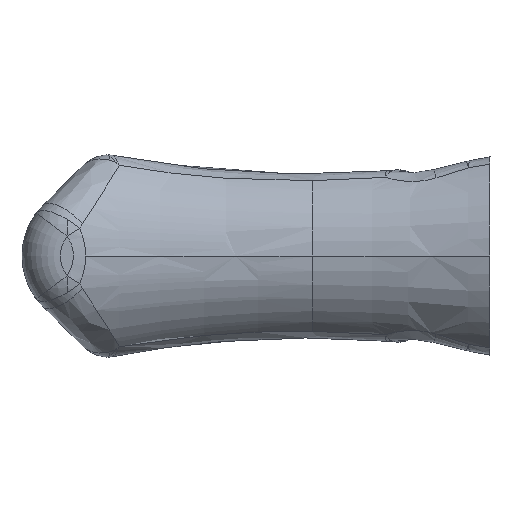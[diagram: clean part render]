
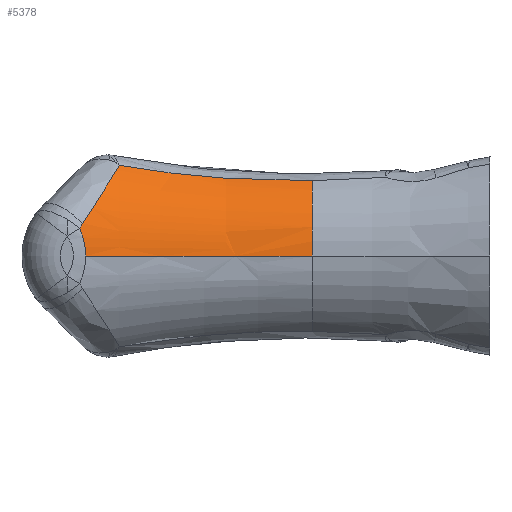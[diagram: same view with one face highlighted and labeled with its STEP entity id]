
A CAD part, left-side view. The second image highlights one B-rep face of the part: STEP entity #5378.
In plain terms, the highlighted toroidal (fillet/blend) face has major radius 208.719 mm and minor radius 185.111 mm.
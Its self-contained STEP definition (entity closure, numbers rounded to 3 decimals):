
#231 = DIRECTION ( 'NONE',  ( -1., 0., 0. ) ) ;
#347 = CARTESIAN_POINT ( 'NONE',  ( -310.696, 64.488, 25.983 ) ) ;
#418 = CARTESIAN_POINT ( 'NONE',  ( -307.871, 63.211, 28.086 ) ) ;
#647 = CARTESIAN_POINT ( 'NONE',  ( -321.046, 73.018, 12.59 ) ) ;
#705 = EDGE_CURVE ( 'NONE', #3358, #5440, #2863, .T. ) ;
#825 = CARTESIAN_POINT ( 'NONE',  ( -313.258, 65.894, 23.695 ) ) ;
#827 = B_SPLINE_CURVE_WITH_KNOTS ( 'NONE', 3,
 ( #3615, #3656, #4132, #1293, #4623, #1784, #5098, #2257 ),
 .UNSPECIFIED., .F., .F.,
 ( 4, 2, 2, 4 ),
 ( 0.011, 0.013, 0.015, 0.019 ),
 .UNSPECIFIED. ) ;
#836 = VERTEX_POINT ( 'NONE', #4522 ) ;
#878 = CARTESIAN_POINT ( 'NONE',  ( -301.785, 17.37, 24.08 ) ) ;
#899 = B_SPLINE_CURVE_WITH_KNOTS ( 'NONE', 3,
 ( #3952, #647, #4912, #2082 ),
 .UNSPECIFIED., .F., .F.,
 ( 4, 4 ),
 ( 0., 0.002 ),
 .UNSPECIFIED. ) ;
#901 = EDGE_CURVE ( 'NONE', #4754, #2436, #4038, .T. ) ;
#1188 = AXIS2_PLACEMENT_3D ( 'NONE', #5919, #3066, #231 ) ;
#1202 = EDGE_LOOP ( 'NONE', ( #6044, #1554, #4836, #1295, #6018, #1652 ) ) ;
#1293 = CARTESIAN_POINT ( 'NONE',  ( -321.548, 72.657, 9.405 ) ) ;
#1295 = ORIENTED_EDGE ( 'NONE', *, *, #901, .T. ) ;
#1296 = CARTESIAN_POINT ( 'NONE',  ( -316.564, 68.248, 19.938 ) ) ;
#1351 = CARTESIAN_POINT ( 'NONE',  ( -302.108, 23.712, 24.165 ) ) ;
#1554 = ORIENTED_EDGE ( 'NONE', *, *, #1622, .T. ) ;
#1561 = AXIS2_PLACEMENT_3D ( 'NONE', #2595, #3996, #5921 ) ;
#1622 = EDGE_CURVE ( 'NONE', #5440, #4441, #2073, .T. ) ;
#1652 = ORIENTED_EDGE ( 'NONE', *, *, #4224, .T. ) ;
#1784 = CARTESIAN_POINT ( 'NONE',  ( -321.638, 72.092, 7.004 ) ) ;
#1786 = CARTESIAN_POINT ( 'NONE',  ( -318.882, 70.421, 16.55 ) ) ;
#1838 = CARTESIAN_POINT ( 'NONE',  ( -302.604, 30.036, 24.392 ) ) ;
#1863 = CARTESIAN_POINT ( 'NONE',  ( -321.66, 71.952, 4.547 ) ) ;
#1895 = CARTESIAN_POINT ( 'NONE',  ( -301.679, 13.135, 24.108 ) ) ;
#2073 = CIRCLE ( 'NONE', #6058, 23.608 ) ;
#2082 = CARTESIAN_POINT ( 'NONE',  ( -321.417, 73.495, 11.706 ) ) ;
#2206 = CARTESIAN_POINT ( 'NONE',  ( -320.842, 72.744, 13.003 ) ) ;
#2257 = CARTESIAN_POINT ( 'NONE',  ( -321.66, 71.952, 4.547 ) ) ;
#2259 = CARTESIAN_POINT ( 'NONE',  ( -320.109, 71.798, 14.437 ) ) ;
#2266 = DIRECTION ( 'NONE',  ( 0., 1., 0. ) ) ;
#2318 = CARTESIAN_POINT ( 'NONE',  ( -303.265, 36.345, 24.763 ) ) ;
#2436 = VERTEX_POINT ( 'NONE', #2206 ) ;
#2595 = CARTESIAN_POINT ( 'NONE',  ( -288.46, 13.135, 4.547 ) ) ;
#2713 = CARTESIAN_POINT ( 'NONE',  ( -308.606, 63.511, 27.589 ) ) ;
#2734 = CARTESIAN_POINT ( 'NONE',  ( -320.842, 72.744, 13.003 ) ) ;
#2783 = CARTESIAN_POINT ( 'NONE',  ( -304.683, 46.784, 25.683 ) ) ;
#2863 = CIRCLE ( 'NONE', #1188, 185.111 ) ;
#2916 = EDGE_CURVE ( 'NONE', #2436, #836, #899, .T. ) ;
#3066 = DIRECTION ( 'NONE',  ( 0., 0., -1. ) ) ;
#3116 = FACE_OUTER_BOUND ( 'NONE', #1202, .T. ) ;
#3120 = CARTESIAN_POINT ( 'NONE',  ( -307.871, 63.211, 28.086 ) ) ;
#3192 = CARTESIAN_POINT ( 'NONE',  ( -309.319, 63.827, 27.068 ) ) ;
#3263 = CARTESIAN_POINT ( 'NONE',  ( -306.952, 59.141, 27.362 ) ) ;
#3315 = EDGE_CURVE ( 'NONE', #4441, #4754, #4394, .T. ) ;
#3358 = VERTEX_POINT ( 'NONE', #1863 ) ;
#3401 = TOROIDAL_SURFACE ( 'NONE', #1561, 208.719, 185.111 ) ;
#3615 = CARTESIAN_POINT ( 'NONE',  ( -321.417, 73.495, 11.706 ) ) ;
#3656 = CARTESIAN_POINT ( 'NONE',  ( -321.454, 73.255, 11.143 ) ) ;
#3658 = CARTESIAN_POINT ( 'NONE',  ( -311.356, 64.831, 25.423 ) ) ;
#3952 = CARTESIAN_POINT ( 'NONE',  ( -320.842, 72.744, 13.003 ) ) ;
#3996 = DIRECTION ( 'NONE',  ( 0., 1., 0. ) ) ;
#4034 = CARTESIAN_POINT ( 'NONE',  ( -312.068, 13.135, 4.547 ) ) ;
#4038 = B_SPLINE_CURVE_WITH_KNOTS ( 'NONE', 3,
 ( #6041, #2713, #3192, #347, #3658, #825, #4135, #1296, #4625, #1786, #5100, #2259, #5585, #2734 ),
 .UNSPECIFIED., .F., .F.,
 ( 4, 2, 2, 2, 2, 2, 4 ),
 ( 0., 0.003, 0.006, 0.012, 0.017, 0.02, 0.023 ),
 .UNSPECIFIED. ) ;
#4132 = CARTESIAN_POINT ( 'NONE',  ( -321.488, 73.038, 10.571 ) ) ;
#4135 = CARTESIAN_POINT ( 'NONE',  ( -314.422, 66.649, 22.479 ) ) ;
#4188 = CARTESIAN_POINT ( 'NONE',  ( -301.981, 21.6, 24.121 ) ) ;
#4224 = EDGE_CURVE ( 'NONE', #836, #3358, #827, .T. ) ;
#4394 = B_SPLINE_CURVE_WITH_KNOTS ( 'NONE', 3,
 ( #4660, #6096, #878, #4188, #1351, #4679, #1838, #5158, #2318, #5641, #2783, #6112, #3263, #418 ),
 .UNSPECIFIED., .F., .F.,
 ( 4, 2, 2, 2, 2, 2, 4 ),
 ( 0.048, 0.055, 0.061, 0.067, 0.074, 0.086, 0.099 ),
 .UNSPECIFIED. ) ;
#4441 = VERTEX_POINT ( 'NONE', #1895 ) ;
#4522 = CARTESIAN_POINT ( 'NONE',  ( -321.417, 73.495, 11.706 ) ) ;
#4623 = CARTESIAN_POINT ( 'NONE',  ( -321.575, 72.491, 8.808 ) ) ;
#4625 = CARTESIAN_POINT ( 'NONE',  ( -317.543, 69.091, 18.612 ) ) ;
#4660 = CARTESIAN_POINT ( 'NONE',  ( -301.679, 13.135, 24.108 ) ) ;
#4679 = CARTESIAN_POINT ( 'NONE',  ( -302.42, 27.93, 24.3 ) ) ;
#4754 = VERTEX_POINT ( 'NONE', #3120 ) ;
#4836 = ORIENTED_EDGE ( 'NONE', *, *, #3315, .T. ) ;
#4912 = CARTESIAN_POINT ( 'NONE',  ( -321.238, 73.267, 12.157 ) ) ;
#5098 = CARTESIAN_POINT ( 'NONE',  ( -321.66, 71.952, 5.785 ) ) ;
#5100 = CARTESIAN_POINT ( 'NONE',  ( -319.307, 70.875, 15.849 ) ) ;
#5109 = CARTESIAN_POINT ( 'NONE',  ( -288.46, 13.135, 4.547 ) ) ;
#5158 = CARTESIAN_POINT ( 'NONE',  ( -303.027, 34.243, 24.623 ) ) ;
#5378 = ADVANCED_FACE ( 'NONE', ( #3116 ), #3401, .F. ) ;
#5440 = VERTEX_POINT ( 'NONE', #4034 ) ;
#5585 = CARTESIAN_POINT ( 'NONE',  ( -320.486, 72.267, 13.723 ) ) ;
#5594 = DIRECTION ( 'NONE',  ( -1., 0., 0. ) ) ;
#5641 = CARTESIAN_POINT ( 'NONE',  ( -304.055, 42.626, 25.256 ) ) ;
#5919 = CARTESIAN_POINT ( 'NONE',  ( -497.179, 13.135, 4.547 ) ) ;
#5921 = DIRECTION ( 'NONE',  ( -1., 0., 0. ) ) ;
#6018 = ORIENTED_EDGE ( 'NONE', *, *, #2916, .T. ) ;
#6041 = CARTESIAN_POINT ( 'NONE',  ( -307.871, 63.211, 28.086 ) ) ;
#6044 = ORIENTED_EDGE ( 'NONE', *, *, #705, .T. ) ;
#6058 = AXIS2_PLACEMENT_3D ( 'NONE', #5109, #2266, #5594 ) ;
#6096 = CARTESIAN_POINT ( 'NONE',  ( -301.716, 15.251, 24.082 ) ) ;
#6112 = CARTESIAN_POINT ( 'NONE',  ( -306.131, 55.041, 26.736 ) ) ;
